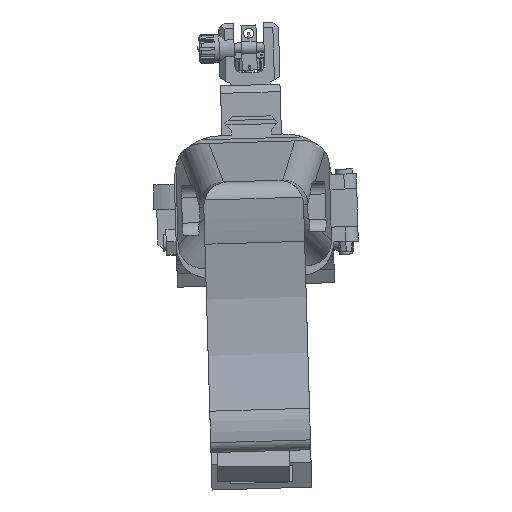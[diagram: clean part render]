
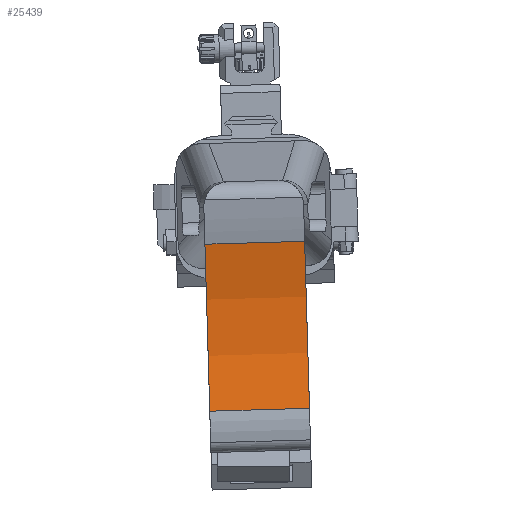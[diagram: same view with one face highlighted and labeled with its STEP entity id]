
A CAD part, left-side view. The second image highlights one B-rep face of the part: STEP entity #25439.
In plain terms, the highlighted cylindrical face has radius 137.628 mm (diameter 275.256 mm), a partial arc.
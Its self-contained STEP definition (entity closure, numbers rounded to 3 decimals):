
#439=CIRCLE('',#27370,137.628);
#440=CIRCLE('',#27371,137.628);
#712=CYLINDRICAL_SURFACE('',#27369,137.628);
#6049=ORIENTED_EDGE('',*,*,#10842,.T.);
#6050=ORIENTED_EDGE('',*,*,#10845,.T.);
#6051=ORIENTED_EDGE('',*,*,#10846,.F.);
#6052=ORIENTED_EDGE('',*,*,#10847,.F.);
#10842=EDGE_CURVE('',#13655,#13654,#16655,.T.);
#10845=EDGE_CURVE('',#13654,#13657,#439,.T.);
#10846=EDGE_CURVE('',#13658,#13657,#16656,.T.);
#10847=EDGE_CURVE('',#13655,#13658,#440,.T.);
#13654=VERTEX_POINT('',#40102);
#13655=VERTEX_POINT('',#40104);
#13657=VERTEX_POINT('',#40113);
#13658=VERTEX_POINT('',#40115);
#16655=LINE('',#40103,#19783);
#16656=LINE('',#40114,#19784);
#19783=VECTOR('',#32686,1000.);
#19784=VECTOR('',#32693,1000.);
#21563=EDGE_LOOP('',(#6049,#6050,#6051,#6052));
#22981=FACE_BOUND('',#21563,.T.);
#25439=ADVANCED_FACE('',(#22981),#712,.F.);
#27369=AXIS2_PLACEMENT_3D('',#40111,#32689,#32690);
#27370=AXIS2_PLACEMENT_3D('',#40112,#32691,#32692);
#27371=AXIS2_PLACEMENT_3D('',#40116,#32694,#32695);
#32686=DIRECTION('',(0.,1.,0.));
#32689=DIRECTION('',(0.,1.,0.));
#32690=DIRECTION('',(0.,0.,1.));
#32691=DIRECTION('',(0.,1.,0.));
#32692=DIRECTION('',(-1.,0.,0.));
#32693=DIRECTION('',(0.,1.,0.));
#32694=DIRECTION('',(0.,1.,0.));
#32695=DIRECTION('',(-1.,0.,0.));
#40102=CARTESIAN_POINT('',(-98.279,20.,67.356));
#40103=CARTESIAN_POINT('',(-98.279,-20.,67.356));
#40104=CARTESIAN_POINT('',(-98.279,-20.,67.356));
#40111=CARTESIAN_POINT('',(-231.77,-20.,33.869));
#40112=CARTESIAN_POINT('',(-231.77,20.,33.869));
#40113=CARTESIAN_POINT('',(-98.279,20.,0.382));
#40114=CARTESIAN_POINT('',(-98.279,-20.,0.382));
#40115=CARTESIAN_POINT('',(-98.279,-20.,0.382));
#40116=CARTESIAN_POINT('',(-231.77,-20.,33.869));
